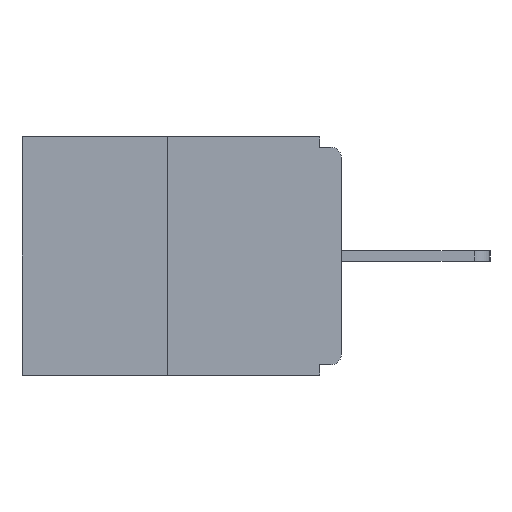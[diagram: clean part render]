
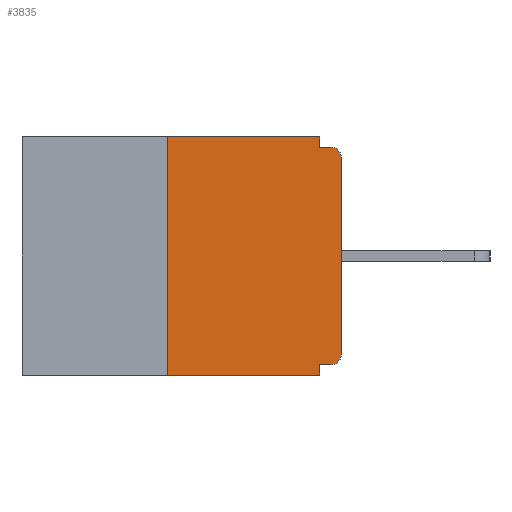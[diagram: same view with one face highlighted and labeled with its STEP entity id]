
A CAD part, left-side view. The second image highlights one B-rep face of the part: STEP entity #3835.
In plain terms, the highlighted planar face has unit normal (-1, 0, 0).
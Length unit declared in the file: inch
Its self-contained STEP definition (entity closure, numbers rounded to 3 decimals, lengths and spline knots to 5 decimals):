
#112 = CARTESIAN_POINT ( 'NONE',  ( 0., 0.031, 0. ) ) ;
#184 = DIRECTION ( 'NONE',  ( 0., -1., 0. ) ) ;
#258 = CARTESIAN_POINT ( 'NONE',  ( 0., 0.46, 0. ) ) ;
#433 = VECTOR ( 'NONE', #12516, 39.37008 ) ;
#512 = CARTESIAN_POINT ( 'NONE',  ( 0., 0.25, -0.343 ) ) ;
#681 = CIRCLE ( 'NONE', #6517, 0.015 ) ;
#1062 = EDGE_CURVE ( 'NONE', #2665, #1425, #4123, .T. ) ;
#1149 = FACE_OUTER_BOUND ( 'NONE', #4155, .T. ) ;
#1190 = CARTESIAN_POINT ( 'NONE',  ( 0., 0., -0.328 ) ) ;
#1241 = ORIENTED_EDGE ( 'NONE', *, *, #9754, .F. ) ;
#1336 = CARTESIAN_POINT ( 'NONE',  ( 0., 0., -0.313 ) ) ;
#1425 = VERTEX_POINT ( 'NONE', #4567 ) ;
#1603 = EDGE_CURVE ( 'NONE', #4335, #11729, #2697, .T. ) ;
#1618 = ORIENTED_EDGE ( 'NONE', *, *, #7796, .T. ) ;
#1901 = CARTESIAN_POINT ( 'NONE',  ( 0., 0.015, -0.328 ) ) ;
#1990 = ORIENTED_EDGE ( 'NONE', *, *, #3405, .F. ) ;
#2019 = CIRCLE ( 'NONE', #13617, 0.015 ) ;
#2419 = DIRECTION ( 'NONE',  ( -1., 0., 0. ) ) ;
#2649 = DIRECTION ( 'NONE',  ( 0., 0., -1. ) ) ;
#2665 = VERTEX_POINT ( 'NONE', #1336 ) ;
#2683 = DIRECTION ( 'NONE',  ( -1., 0., 0. ) ) ;
#2697 = LINE ( 'NONE', #112, #5398 ) ;
#2700 = CARTESIAN_POINT ( 'NONE',  ( 0., 0.015, -0.313 ) ) ;
#3288 = CARTESIAN_POINT ( 'NONE',  ( 0., 0.015, -0.015 ) ) ;
#3390 = EDGE_CURVE ( 'NONE', #9823, #4335, #4226, .T. ) ;
#3405 = EDGE_CURVE ( 'NONE', #11729, #13338, #13126, .T. ) ;
#3580 = AXIS2_PLACEMENT_3D ( 'NONE', #11931, #14392, #14313 ) ;
#3835 = ADVANCED_FACE ( 'NONE', ( #1149 ), #11933, .F. ) ;
#3948 = ORIENTED_EDGE ( 'NONE', *, *, #3390, .F. ) ;
#4123 = LINE ( 'NONE', #7536, #6504 ) ;
#4155 = EDGE_LOOP ( 'NONE', ( #3948, #7063, #12860, #1241, #7443, #1618, #10652, #13528, #1990, #8131 ) ) ;
#4226 = LINE ( 'NONE', #258, #10253 ) ;
#4335 = VERTEX_POINT ( 'NONE', #11553 ) ;
#4450 = CARTESIAN_POINT ( 'NONE',  ( 0., 0.031, -0.343 ) ) ;
#4567 = CARTESIAN_POINT ( 'NONE',  ( 0., 0., -0.03 ) ) ;
#4739 = CARTESIAN_POINT ( 'NONE',  ( 0., 0.031, -0.328 ) ) ;
#4779 = VECTOR ( 'NONE', #7749, 39.37008 ) ;
#5057 = VERTEX_POINT ( 'NONE', #4739 ) ;
#5398 = VECTOR ( 'NONE', #7857, 39.37008 ) ;
#5477 = VECTOR ( 'NONE', #9627, 39.37008 ) ;
#5540 = LINE ( 'NONE', #6570, #4779 ) ;
#5549 = CARTESIAN_POINT ( 'NONE',  ( 0., 0.25, 0. ) ) ;
#5758 = CARTESIAN_POINT ( 'NONE',  ( 0., 0.031, -0.015 ) ) ;
#5943 = EDGE_CURVE ( 'NONE', #14091, #9823, #14275, .T. ) ;
#6504 = VECTOR ( 'NONE', #6968, 39.37008 ) ;
#6517 = AXIS2_PLACEMENT_3D ( 'NONE', #2700, #2683, #2649 ) ;
#6570 = CARTESIAN_POINT ( 'NONE',  ( 0., 0.031, -0.343 ) ) ;
#6968 = DIRECTION ( 'NONE',  ( 0., 0., 1. ) ) ;
#7063 = ORIENTED_EDGE ( 'NONE', *, *, #5943, .F. ) ;
#7443 = ORIENTED_EDGE ( 'NONE', *, *, #12356, .F. ) ;
#7536 = CARTESIAN_POINT ( 'NONE',  ( 0., 0., 0. ) ) ;
#7749 = DIRECTION ( 'NONE',  ( 0., 0., -1. ) ) ;
#7796 = EDGE_CURVE ( 'NONE', #13200, #2665, #681, .T. ) ;
#7857 = DIRECTION ( 'NONE',  ( 0., 0., -1. ) ) ;
#8131 = ORIENTED_EDGE ( 'NONE', *, *, #1603, .F. ) ;
#8522 = LINE ( 'NONE', #1190, #11365 ) ;
#8765 = EDGE_CURVE ( 'NONE', #14091, #10365, #9986, .T. ) ;
#9240 = DIRECTION ( 'NONE',  ( 0., 1., 0. ) ) ;
#9286 = CARTESIAN_POINT ( 'NONE',  ( 0., 0.015, -0.03 ) ) ;
#9627 = DIRECTION ( 'NONE',  ( 0., 0., 1. ) ) ;
#9754 = EDGE_CURVE ( 'NONE', #5057, #10365, #5540, .T. ) ;
#9762 = CARTESIAN_POINT ( 'NONE',  ( 0., 0.25, 0. ) ) ;
#9823 = VERTEX_POINT ( 'NONE', #5549 ) ;
#9986 = LINE ( 'NONE', #14610, #433 ) ;
#10253 = VECTOR ( 'NONE', #184, 39.37008 ) ;
#10335 = DIRECTION ( 'NONE',  ( 0., 0., -1. ) ) ;
#10365 = VERTEX_POINT ( 'NONE', #4450 ) ;
#10652 = ORIENTED_EDGE ( 'NONE', *, *, #1062, .T. ) ;
#10919 = CARTESIAN_POINT ( 'NONE',  ( 0., 0., -0.015 ) ) ;
#11365 = VECTOR ( 'NONE', #9240, 39.37008 ) ;
#11553 = CARTESIAN_POINT ( 'NONE',  ( 0., 0.031, 0. ) ) ;
#11729 = VERTEX_POINT ( 'NONE', #5758 ) ;
#11931 = CARTESIAN_POINT ( 'NONE',  ( 0., 0.46, 0. ) ) ;
#11933 = PLANE ( 'NONE',  #3580 ) ;
#12356 = EDGE_CURVE ( 'NONE', #13200, #5057, #8522, .T. ) ;
#12376 = EDGE_CURVE ( 'NONE', #1425, #13338, #2019, .T. ) ;
#12516 = DIRECTION ( 'NONE',  ( 0., -1., 0. ) ) ;
#12798 = VECTOR ( 'NONE', #14439, 39.37008 ) ;
#12860 = ORIENTED_EDGE ( 'NONE', *, *, #8765, .T. ) ;
#13126 = LINE ( 'NONE', #10919, #12798 ) ;
#13200 = VERTEX_POINT ( 'NONE', #1901 ) ;
#13338 = VERTEX_POINT ( 'NONE', #3288 ) ;
#13528 = ORIENTED_EDGE ( 'NONE', *, *, #12376, .T. ) ;
#13617 = AXIS2_PLACEMENT_3D ( 'NONE', #9286, #2419, #10335 ) ;
#14091 = VERTEX_POINT ( 'NONE', #512 ) ;
#14275 = LINE ( 'NONE', #9762, #5477 ) ;
#14313 = DIRECTION ( 'NONE',  ( 0., 0., -1. ) ) ;
#14392 = DIRECTION ( 'NONE',  ( 1., 0., 0. ) ) ;
#14439 = DIRECTION ( 'NONE',  ( 0., -1., 0. ) ) ;
#14610 = CARTESIAN_POINT ( 'NONE',  ( 0., 0.46, -0.343 ) ) ;
